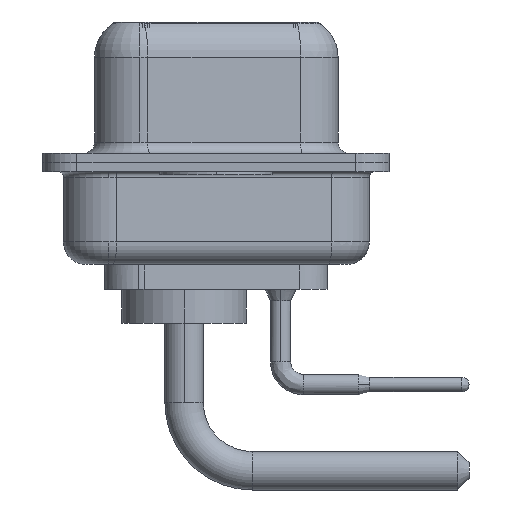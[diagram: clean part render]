
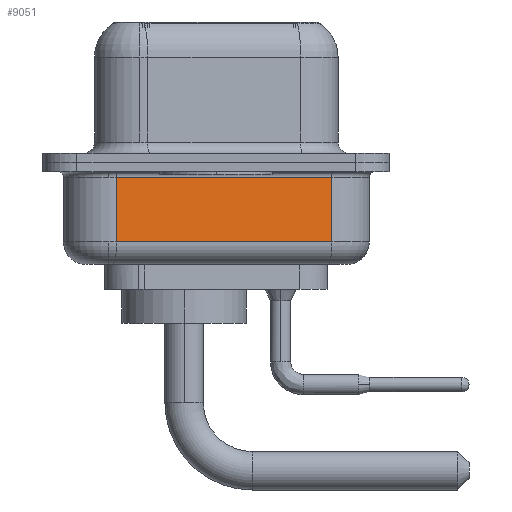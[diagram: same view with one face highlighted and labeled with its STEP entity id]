
A CAD part, left-side view. The second image highlights one B-rep face of the part: STEP entity #9051.
In plain terms, the highlighted planar face has unit normal (-0.985, -0.174, 0).
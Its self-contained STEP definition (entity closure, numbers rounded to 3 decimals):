
#76 = DIRECTION ( 'NONE',  ( 0.985, 0.174, 0. ) ) ;
#406 = EDGE_CURVE ( 'NONE', #965, #3462, #8464, .T. ) ;
#581 = ORIENTED_EDGE ( 'NONE', *, *, #8361, .T. ) ;
#630 = EDGE_CURVE ( 'NONE', #965, #15982, #8760, .T. ) ;
#965 = VERTEX_POINT ( 'NONE', #2383 ) ;
#1847 = ORIENTED_EDGE ( 'NONE', *, *, #14741, .T. ) ;
#2383 = CARTESIAN_POINT ( 'NONE',  ( 2.93, 4.403, -3.5 ) ) ;
#2701 = EDGE_LOOP ( 'NONE', ( #4117, #2956, #1847, #581 ) ) ;
#2956 = ORIENTED_EDGE ( 'NONE', *, *, #630, .T. ) ;
#3462 = VERTEX_POINT ( 'NONE', #17930 ) ;
#3772 = CARTESIAN_POINT ( 'NONE',  ( 2.93, 4.403, -0.65 ) ) ;
#4117 = ORIENTED_EDGE ( 'NONE', *, *, #406, .F. ) ;
#5397 = VECTOR ( 'NONE', #17740, 1000. ) ;
#6572 = LINE ( 'NONE', #10996, #16219 ) ;
#7295 = CARTESIAN_POINT ( 'NONE',  ( 4.605, -5.097, -0.65 ) ) ;
#7596 = FACE_OUTER_BOUND ( 'NONE', #2701, .T. ) ;
#8361 = EDGE_CURVE ( 'NONE', #16020, #3462, #9907, .T. ) ;
#8464 = LINE ( 'NONE', #17167, #10739 ) ;
#8760 = LINE ( 'NONE', #14627, #5397 ) ;
#9051 = ADVANCED_FACE ( 'NONE', ( #7596 ), #16409, .F. ) ;
#9907 = LINE ( 'NONE', #3772, #16552 ) ;
#10739 = VECTOR ( 'NONE', #15896, 1000. ) ;
#10996 = CARTESIAN_POINT ( 'NONE',  ( 4.605, -5.097, -4.5 ) ) ;
#12211 = DIRECTION ( 'NONE',  ( -0.174, 0.985, 0. ) ) ;
#13494 = CARTESIAN_POINT ( 'NONE',  ( 2.93, 4.403, -4.5 ) ) ;
#14627 = CARTESIAN_POINT ( 'NONE',  ( 2.93, 4.403, -3.5 ) ) ;
#14741 = EDGE_CURVE ( 'NONE', #15982, #16020, #6572, .T. ) ;
#15301 = DIRECTION ( 'NONE',  ( 0., 0., 1. ) ) ;
#15666 = DIRECTION ( 'NONE',  ( -0.174, 0.985, 0. ) ) ;
#15896 = DIRECTION ( 'NONE',  ( 0., 0., 1. ) ) ;
#15982 = VERTEX_POINT ( 'NONE', #19041 ) ;
#16020 = VERTEX_POINT ( 'NONE', #7295 ) ;
#16219 = VECTOR ( 'NONE', #15301, 1000. ) ;
#16409 = PLANE ( 'NONE',  #16984 ) ;
#16552 = VECTOR ( 'NONE', #15666, 1000. ) ;
#16984 = AXIS2_PLACEMENT_3D ( 'NONE', #13494, #76, #12211 ) ;
#17167 = CARTESIAN_POINT ( 'NONE',  ( 2.93, 4.403, -4.5 ) ) ;
#17740 = DIRECTION ( 'NONE',  ( 0.174, -0.985, 0. ) ) ;
#17930 = CARTESIAN_POINT ( 'NONE',  ( 2.93, 4.403, -0.65 ) ) ;
#19041 = CARTESIAN_POINT ( 'NONE',  ( 4.605, -5.097, -3.5 ) ) ;
